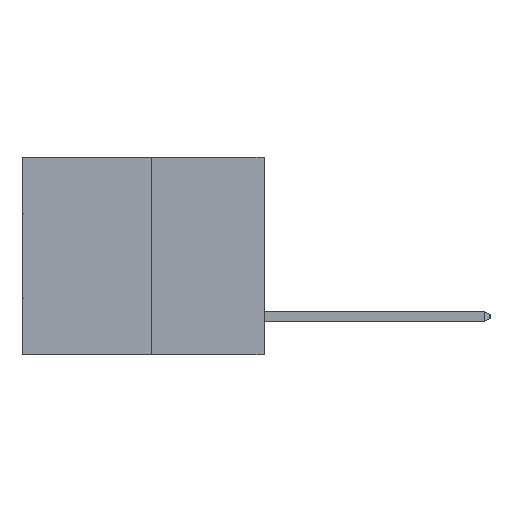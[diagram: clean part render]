
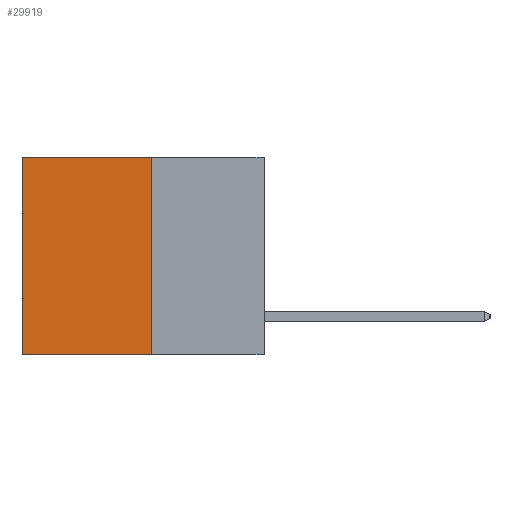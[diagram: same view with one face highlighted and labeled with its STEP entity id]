
A CAD part, left-side view. The second image highlights one B-rep face of the part: STEP entity #29919.
In plain terms, the highlighted planar face has unit normal (-1, 0, 0).
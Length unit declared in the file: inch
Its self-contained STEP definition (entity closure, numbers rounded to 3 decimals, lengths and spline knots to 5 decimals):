
#465 = VERTEX_POINT ( 'NONE', #6585 ) ;
#979 = ORIENTED_EDGE ( 'NONE', *, *, #24207, .T. ) ;
#1866 = DIRECTION ( 'NONE',  ( 0., 0., -1. ) ) ;
#2373 = DIRECTION ( 'NONE',  ( 0., 1., 0. ) ) ;
#2601 = VECTOR ( 'NONE', #25834, 39.37008 ) ;
#3258 = FACE_OUTER_BOUND ( 'NONE', #18803, .T. ) ;
#3524 = CARTESIAN_POINT ( 'NONE',  ( 0.3165, 0.28, -0.49 ) ) ;
#3738 = DIRECTION ( 'NONE',  ( 0., 0., -1. ) ) ;
#3949 = LINE ( 'NONE', #6326, #15776 ) ;
#6326 = CARTESIAN_POINT ( 'NONE',  ( 0.3165, 0.6, -0.49 ) ) ;
#6585 = CARTESIAN_POINT ( 'NONE',  ( 0.3165, 0.6, -0.49 ) ) ;
#7233 = ORIENTED_EDGE ( 'NONE', *, *, #16737, .F. ) ;
#7549 = CARTESIAN_POINT ( 'NONE',  ( 0.3165, 0.28, 0. ) ) ;
#8922 = CARTESIAN_POINT ( 'NONE',  ( 0.3165, 0.28, -0.49 ) ) ;
#9325 = LINE ( 'NONE', #11229, #12614 ) ;
#10193 = EDGE_CURVE ( 'NONE', #26156, #465, #14660, .T. ) ;
#11229 = CARTESIAN_POINT ( 'NONE',  ( 0.3165, 0.28, -0.49 ) ) ;
#12614 = VECTOR ( 'NONE', #3738, 39.37008 ) ;
#13422 = PLANE ( 'NONE',  #18603 ) ;
#14660 = LINE ( 'NONE', #25769, #20919 ) ;
#14679 = ORIENTED_EDGE ( 'NONE', *, *, #10193, .F. ) ;
#15776 = VECTOR ( 'NONE', #22838, 39.37008 ) ;
#16737 = EDGE_CURVE ( 'NONE', #19910, #26156, #9325, .T. ) ;
#18603 = AXIS2_PLACEMENT_3D ( 'NONE', #3524, #20010, #1866 ) ;
#18803 = EDGE_LOOP ( 'NONE', ( #22705, #14679, #7233, #979 ) ) ;
#19910 = VERTEX_POINT ( 'NONE', #7549 ) ;
#20010 = DIRECTION ( 'NONE',  ( 1., 0., 0. ) ) ;
#20697 = LINE ( 'NONE', #23579, #2601 ) ;
#20919 = VECTOR ( 'NONE', #2373, 39.37008 ) ;
#22705 = ORIENTED_EDGE ( 'NONE', *, *, #26215, .T. ) ;
#22838 = DIRECTION ( 'NONE',  ( 0., 0., -1. ) ) ;
#23520 = VERTEX_POINT ( 'NONE', #29381 ) ;
#23579 = CARTESIAN_POINT ( 'NONE',  ( 0.3165, 0.28, 0. ) ) ;
#24207 = EDGE_CURVE ( 'NONE', #19910, #23520, #20697, .T. ) ;
#25769 = CARTESIAN_POINT ( 'NONE',  ( 0.3165, 0.28, -0.49 ) ) ;
#25834 = DIRECTION ( 'NONE',  ( 0., 1., 0. ) ) ;
#26156 = VERTEX_POINT ( 'NONE', #8922 ) ;
#26215 = EDGE_CURVE ( 'NONE', #23520, #465, #3949, .T. ) ;
#29381 = CARTESIAN_POINT ( 'NONE',  ( 0.3165, 0.6, 0. ) ) ;
#29919 = ADVANCED_FACE ( 'NONE', ( #3258 ), #13422, .F. ) ;
